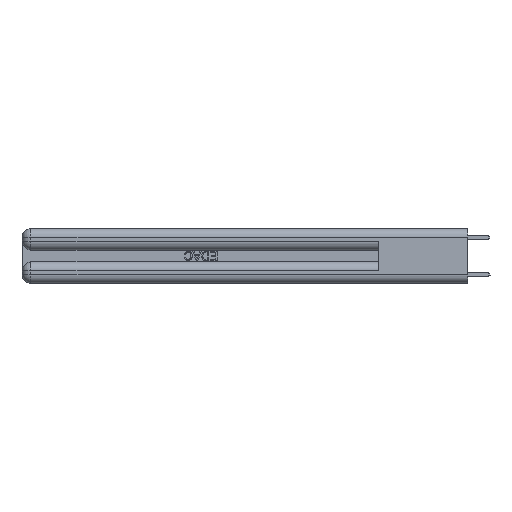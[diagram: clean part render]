
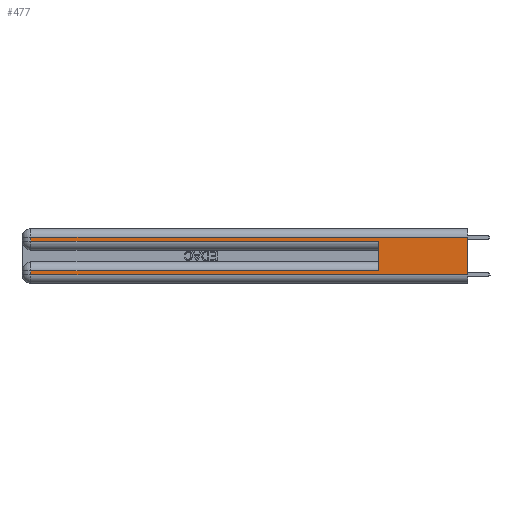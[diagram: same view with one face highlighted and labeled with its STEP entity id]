
A CAD part, left-side view. The second image highlights one B-rep face of the part: STEP entity #477.
In plain terms, the highlighted planar face has unit normal (-1, 0, 0).
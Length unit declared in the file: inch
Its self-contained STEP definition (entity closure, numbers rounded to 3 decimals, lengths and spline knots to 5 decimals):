
#28 = FACE_OUTER_BOUND ( 'NONE', #13669, .T. ) ;
#477 = ADVANCED_FACE ( 'NONE', ( #28 ), #19803, .F. ) ;
#529 = VERTEX_POINT ( 'NONE', #27137 ) ;
#1596 = DIRECTION ( 'NONE',  ( 0., 1., 0. ) ) ;
#1651 = CARTESIAN_POINT ( 'NONE',  ( 0., 0.6, 0.285 ) ) ;
#1770 = CARTESIAN_POINT ( 'NONE',  ( 0., 0., 0.285 ) ) ;
#2390 = CARTESIAN_POINT ( 'NONE',  ( 0., 2.94, 0.285 ) ) ;
#2738 = DIRECTION ( 'NONE',  ( 0., 0., -1. ) ) ;
#3064 = LINE ( 'NONE', #22375, #21761 ) ;
#3232 = LINE ( 'NONE', #27490, #30770 ) ;
#3380 = ORIENTED_EDGE ( 'NONE', *, *, #4497, .T. ) ;
#3671 = VERTEX_POINT ( 'NONE', #29037 ) ;
#3857 = VERTEX_POINT ( 'NONE', #2390 ) ;
#4497 = EDGE_CURVE ( 'NONE', #16571, #10790, #30558, .T. ) ;
#4641 = CARTESIAN_POINT ( 'NONE',  ( 0., 2.94, 0.06 ) ) ;
#5115 = EDGE_CURVE ( 'NONE', #9403, #3857, #3064, .T. ) ;
#5606 = DIRECTION ( 'NONE',  ( 0., 0., -1. ) ) ;
#6100 = ORIENTED_EDGE ( 'NONE', *, *, #25840, .T. ) ;
#6545 = EDGE_CURVE ( 'NONE', #529, #10790, #27473, .T. ) ;
#7159 = CARTESIAN_POINT ( 'NONE',  ( 0., 2.94, 0.37 ) ) ;
#7484 = ORIENTED_EDGE ( 'NONE', *, *, #10107, .F. ) ;
#8774 = VERTEX_POINT ( 'NONE', #1651 ) ;
#9403 = VERTEX_POINT ( 'NONE', #28739 ) ;
#9545 = ORIENTED_EDGE ( 'NONE', *, *, #28103, .T. ) ;
#9700 = VERTEX_POINT ( 'NONE', #27058 ) ;
#10107 = EDGE_CURVE ( 'NONE', #9700, #8774, #25093, .T. ) ;
#10790 = VERTEX_POINT ( 'NONE', #29844 ) ;
#11195 = CARTESIAN_POINT ( 'NONE',  ( 0., 0., 0.31 ) ) ;
#11201 = VECTOR ( 'NONE', #25252, 39.37008 ) ;
#11811 = LINE ( 'NONE', #7159, #13765 ) ;
#13669 = EDGE_LOOP ( 'NONE', ( #14934, #6100, #30851, #21156, #7484, #26450, #9545, #3380 ) ) ;
#13765 = VECTOR ( 'NONE', #21533, 39.37008 ) ;
#14556 = CARTESIAN_POINT ( 'NONE',  ( 0., 0., 0.37 ) ) ;
#14934 = ORIENTED_EDGE ( 'NONE', *, *, #6545, .F. ) ;
#14962 = EDGE_CURVE ( 'NONE', #9700, #3671, #3232, .T. ) ;
#16544 = VECTOR ( 'NONE', #21079, 39.37008 ) ;
#16571 = VERTEX_POINT ( 'NONE', #4641 ) ;
#19274 = VECTOR ( 'NONE', #5606, 39.37008 ) ;
#19803 = PLANE ( 'NONE',  #25302 ) ;
#20107 = EDGE_CURVE ( 'NONE', #3857, #8774, #23476, .T. ) ;
#20985 = DIRECTION ( 'NONE',  ( 0., -1., 0. ) ) ;
#21079 = DIRECTION ( 'NONE',  ( 0., -1., 0. ) ) ;
#21156 = ORIENTED_EDGE ( 'NONE', *, *, #20107, .T. ) ;
#21533 = DIRECTION ( 'NONE',  ( 0., 0., -1. ) ) ;
#21761 = VECTOR ( 'NONE', #24922, 39.37008 ) ;
#22357 = DIRECTION ( 'NONE',  ( 1., 0., 0. ) ) ;
#22375 = CARTESIAN_POINT ( 'NONE',  ( 0., 2.94, 0.37 ) ) ;
#22706 = DIRECTION ( 'NONE',  ( 0., 1., 0. ) ) ;
#23220 = CARTESIAN_POINT ( 'NONE',  ( 0., 0., 0.06 ) ) ;
#23476 = LINE ( 'NONE', #1770, #16544 ) ;
#24922 = DIRECTION ( 'NONE',  ( 0., 0., -1. ) ) ;
#25093 = LINE ( 'NONE', #30349, #11201 ) ;
#25252 = DIRECTION ( 'NONE',  ( 0., 0., 1. ) ) ;
#25302 = AXIS2_PLACEMENT_3D ( 'NONE', #14556, #22357, #2738 ) ;
#25840 = EDGE_CURVE ( 'NONE', #529, #9403, #28886, .T. ) ;
#26450 = ORIENTED_EDGE ( 'NONE', *, *, #14962, .T. ) ;
#26748 = VECTOR ( 'NONE', #20985, 39.37008 ) ;
#27058 = CARTESIAN_POINT ( 'NONE',  ( 0., 0.6, 0.085 ) ) ;
#27137 = CARTESIAN_POINT ( 'NONE',  ( 0., 0., 0.31 ) ) ;
#27473 = LINE ( 'NONE', #30338, #19274 ) ;
#27490 = CARTESIAN_POINT ( 'NONE',  ( 0., 0., 0.085 ) ) ;
#27910 = VECTOR ( 'NONE', #1596, 39.37008 ) ;
#28103 = EDGE_CURVE ( 'NONE', #3671, #16571, #11811, .T. ) ;
#28739 = CARTESIAN_POINT ( 'NONE',  ( 0., 2.94, 0.31 ) ) ;
#28886 = LINE ( 'NONE', #11195, #27910 ) ;
#29037 = CARTESIAN_POINT ( 'NONE',  ( 0., 2.94, 0.085 ) ) ;
#29844 = CARTESIAN_POINT ( 'NONE',  ( 0., 0., 0.06 ) ) ;
#30338 = CARTESIAN_POINT ( 'NONE',  ( 0., 0., 0.37 ) ) ;
#30349 = CARTESIAN_POINT ( 'NONE',  ( 0., 0.6, 0.145 ) ) ;
#30558 = LINE ( 'NONE', #23220, #26748 ) ;
#30770 = VECTOR ( 'NONE', #22706, 39.37008 ) ;
#30851 = ORIENTED_EDGE ( 'NONE', *, *, #5115, .T. ) ;
